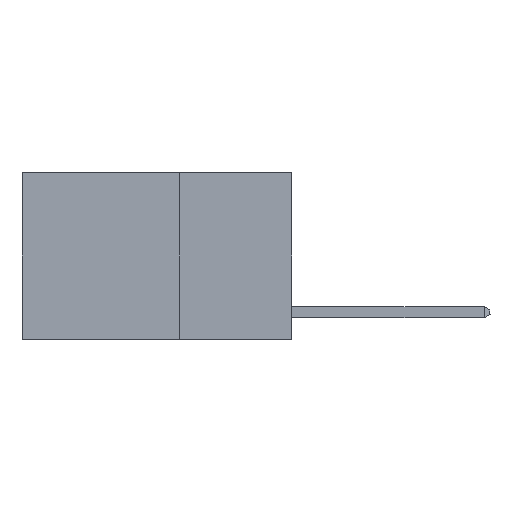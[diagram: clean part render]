
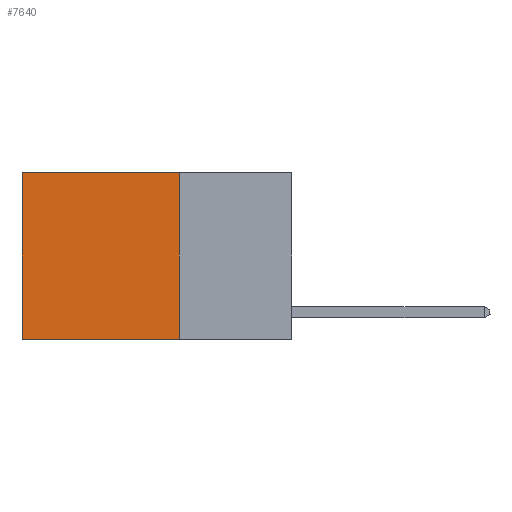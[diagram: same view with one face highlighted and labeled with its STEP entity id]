
A CAD part, left-side view. The second image highlights one B-rep face of the part: STEP entity #7640.
In plain terms, the highlighted planar face has unit normal (-1, 0, 0).
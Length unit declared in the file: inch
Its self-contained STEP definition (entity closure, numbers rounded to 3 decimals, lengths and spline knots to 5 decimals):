
#16 = CARTESIAN_POINT ( 'NONE',  ( 0.2625, 0.25, 0. ) ) ;
#122 = EDGE_CURVE ( 'NONE', #1073, #15056, #11030, .T. ) ;
#499 = CARTESIAN_POINT ( 'NONE',  ( 0.2625, 0.25, -0.37 ) ) ;
#797 = CARTESIAN_POINT ( 'NONE',  ( 0.2625, 0.25, 0. ) ) ;
#847 = DIRECTION ( 'NONE',  ( 0., 0., -1. ) ) ;
#1073 = VERTEX_POINT ( 'NONE', #499 ) ;
#3198 = CARTESIAN_POINT ( 'NONE',  ( 0.2625, 0.25, 0. ) ) ;
#3471 = EDGE_CURVE ( 'NONE', #24474, #10508, #17056, .T. ) ;
#4131 = ORIENTED_EDGE ( 'NONE', *, *, #122, .F. ) ;
#4325 = DIRECTION ( 'NONE',  ( 0., 0., -1. ) ) ;
#5761 = EDGE_CURVE ( 'NONE', #10508, #15056, #12186, .T. ) ;
#5973 = EDGE_CURVE ( 'NONE', #24474, #1073, #10388, .T. ) ;
#6490 = CARTESIAN_POINT ( 'NONE',  ( 0.2625, 0.25, 0. ) ) ;
#7640 = ADVANCED_FACE ( 'NONE', ( #20348 ), #20235, .F. ) ;
#8914 = DIRECTION ( 'NONE',  ( 0., 1., 0. ) ) ;
#9643 = CARTESIAN_POINT ( 'NONE',  ( 0.2625, 0.6, -0.37 ) ) ;
#10010 = ORIENTED_EDGE ( 'NONE', *, *, #3471, .T. ) ;
#10388 = LINE ( 'NONE', #797, #17520 ) ;
#10508 = VERTEX_POINT ( 'NONE', #17643 ) ;
#11030 = LINE ( 'NONE', #16344, #16832 ) ;
#12186 = LINE ( 'NONE', #17895, #22251 ) ;
#15056 = VERTEX_POINT ( 'NONE', #9643 ) ;
#16344 = CARTESIAN_POINT ( 'NONE',  ( 0.2625, 0.25, -0.37 ) ) ;
#16680 = ORIENTED_EDGE ( 'NONE', *, *, #5761, .T. ) ;
#16832 = VECTOR ( 'NONE', #8914, 39.37008 ) ;
#17056 = LINE ( 'NONE', #16, #18120 ) ;
#17435 = DIRECTION ( 'NONE',  ( 0., 1., 0. ) ) ;
#17520 = VECTOR ( 'NONE', #4325, 39.37008 ) ;
#17643 = CARTESIAN_POINT ( 'NONE',  ( 0.2625, 0.6, 0. ) ) ;
#17895 = CARTESIAN_POINT ( 'NONE',  ( 0.2625, 0.6, 0. ) ) ;
#18120 = VECTOR ( 'NONE', #17435, 39.37008 ) ;
#18352 = DIRECTION ( 'NONE',  ( 1., 0., 0. ) ) ;
#20235 = PLANE ( 'NONE',  #21541 ) ;
#20348 = FACE_OUTER_BOUND ( 'NONE', #20741, .T. ) ;
#20423 = ORIENTED_EDGE ( 'NONE', *, *, #5973, .F. ) ;
#20472 = DIRECTION ( 'NONE',  ( 0., 0., -1. ) ) ;
#20741 = EDGE_LOOP ( 'NONE', ( #16680, #4131, #20423, #10010 ) ) ;
#21541 = AXIS2_PLACEMENT_3D ( 'NONE', #3198, #18352, #20472 ) ;
#22251 = VECTOR ( 'NONE', #847, 39.37008 ) ;
#24474 = VERTEX_POINT ( 'NONE', #6490 ) ;
